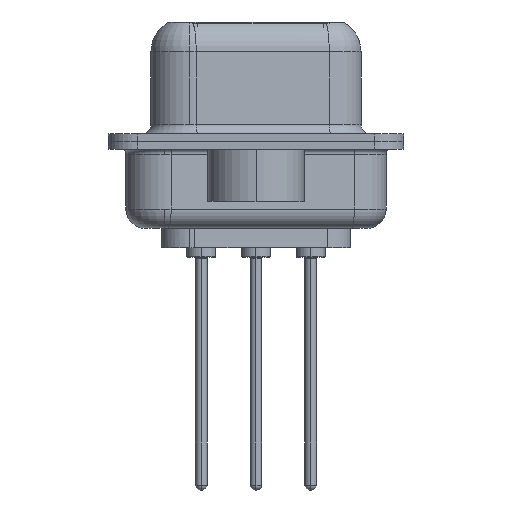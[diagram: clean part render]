
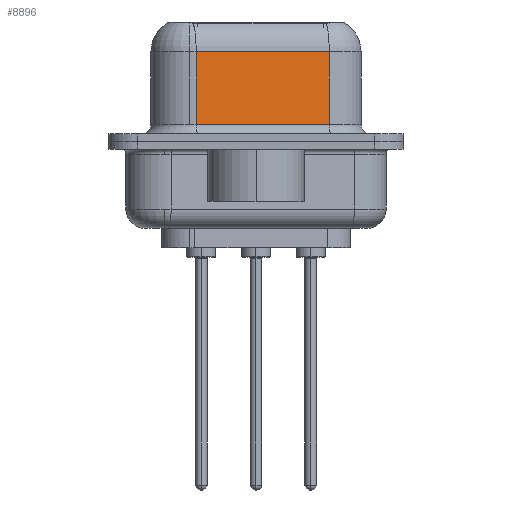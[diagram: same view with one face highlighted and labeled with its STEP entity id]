
A CAD part, left-side view. The second image highlights one B-rep face of the part: STEP entity #8896.
In plain terms, the highlighted planar face has unit normal (-0.985, -0.174, 0).
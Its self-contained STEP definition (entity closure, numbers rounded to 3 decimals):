
#1936 = AXIS2_PLACEMENT_3D ( 'NONE', #27456, #4573, #30283 ) ;
#2017 = VECTOR ( 'NONE', #16795, 1000. ) ;
#2055 = EDGE_CURVE ( 'NONE', #15459, #8599, #31249, .T. ) ;
#4414 = DIRECTION ( 'NONE',  ( 0., 0., -1. ) ) ;
#4573 = DIRECTION ( 'NONE',  ( 0.985, 0.174, 0. ) ) ;
#4576 = LINE ( 'NONE', #24490, #19683 ) ;
#6068 = VECTOR ( 'NONE', #21243, 1000. ) ;
#6681 = EDGE_CURVE ( 'NONE', #8599, #30943, #32426, .T. ) ;
#7797 = LINE ( 'NONE', #25332, #21889 ) ;
#8056 = ORIENTED_EDGE ( 'NONE', *, *, #15651, .F. ) ;
#8409 = CARTESIAN_POINT ( 'NONE',  ( 4.43, 3.103, 6.4 ) ) ;
#8599 = VERTEX_POINT ( 'NONE', #30648 ) ;
#8896 = ADVANCED_FACE ( 'NONE', ( #22307 ), #32451, .F. ) ;
#9818 = ORIENTED_EDGE ( 'NONE', *, *, #27208, .T. ) ;
#12477 = CARTESIAN_POINT ( 'NONE',  ( 5.647, -3.797, 4.65 ) ) ;
#14359 = VERTEX_POINT ( 'NONE', #12477 ) ;
#14407 = ORIENTED_EDGE ( 'NONE', *, *, #2055, .T. ) ;
#15459 = VERTEX_POINT ( 'NONE', #26471 ) ;
#15651 = EDGE_CURVE ( 'NONE', #14359, #30943, #4576, .T. ) ;
#16277 = EDGE_LOOP ( 'NONE', ( #8056, #9818, #14407, #25495 ) ) ;
#16795 = DIRECTION ( 'NONE',  ( 0.174, -0.985, 0. ) ) ;
#19683 = VECTOR ( 'NONE', #4414, 1000. ) ;
#21243 = DIRECTION ( 'NONE',  ( 0., 0., -1. ) ) ;
#21889 = VECTOR ( 'NONE', #27807, 1000. ) ;
#22307 = FACE_OUTER_BOUND ( 'NONE', #16277, .T. ) ;
#24490 = CARTESIAN_POINT ( 'NONE',  ( 5.647, -3.797, 6.4 ) ) ;
#25332 = CARTESIAN_POINT ( 'NONE',  ( 5.647, -3.797, 4.65 ) ) ;
#25495 = ORIENTED_EDGE ( 'NONE', *, *, #6681, .T. ) ;
#26471 = CARTESIAN_POINT ( 'NONE',  ( 4.43, 3.103, 4.65 ) ) ;
#27208 = EDGE_CURVE ( 'NONE', #14359, #15459, #7797, .T. ) ;
#27456 = CARTESIAN_POINT ( 'NONE',  ( 5.647, -3.797, 6.4 ) ) ;
#27807 = DIRECTION ( 'NONE',  ( -0.174, 0.985, 0. ) ) ;
#28191 = CARTESIAN_POINT ( 'NONE',  ( 5.647, -3.797, 0.9 ) ) ;
#29923 = CARTESIAN_POINT ( 'NONE',  ( 5.647, -3.797, 0.9 ) ) ;
#30283 = DIRECTION ( 'NONE',  ( -0.174, 0.985, 0. ) ) ;
#30648 = CARTESIAN_POINT ( 'NONE',  ( 4.43, 3.103, 0.9 ) ) ;
#30943 = VERTEX_POINT ( 'NONE', #28191 ) ;
#31249 = LINE ( 'NONE', #8409, #6068 ) ;
#32426 = LINE ( 'NONE', #29923, #2017 ) ;
#32451 = PLANE ( 'NONE',  #1936 ) ;
